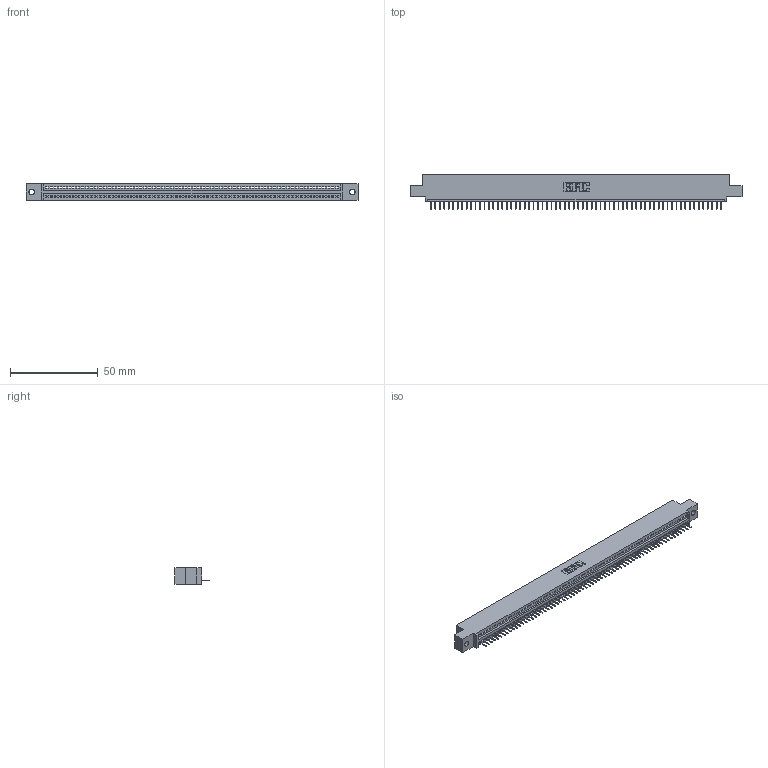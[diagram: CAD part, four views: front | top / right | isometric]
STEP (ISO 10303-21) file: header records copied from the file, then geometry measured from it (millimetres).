
FILE_DESCRIPTION (( 'STEP AP203' ), '1' );
FILE_NAME ('395-066-524-402.STEP', '2019-10-25T08:10:47', ( '' ), ( '' ), 'SwSTEP 2.0', 'SolidWorks 2016', '' );
FILE_SCHEMA (( 'CONFIG_CONTROL_DESIGN' ));
Length unit declared in the file: inch
Products named in the file (3): 395-066-524-402; 345 Part_0.110 Offset - 0.128 Dia; 345-292-001_345-293-124
Assembly tree (67 placements, depth 2):
  395-066-524-402
    345 Part_0.110 Offset - 0.128 Dia
    345-292-001_345-293-124  x66
Bounding box: 188.85 x 19.35 x 9.4 mm (x, y, z)
Volume: 17762.9 mm3; surface area: 22908.2 mm2
Topology: 67 solids, 67 shells, 4222 faces, 12233 edges, 7890 vertices
Faces by surface type: plane 3120, cylinder 1102
Entity records: 46651 total; most frequent: ORIENTED_EDGE 8086, CARTESIAN_POINT 8086, DIRECTION 7027, EDGE_CURVE 4043, LINE 3651, VECTOR 3651, VERTEX_POINT 2690, AXIS2_PLACEMENT_3D 1688
